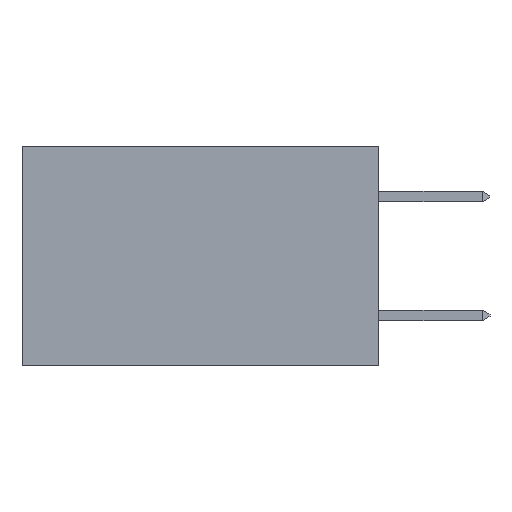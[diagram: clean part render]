
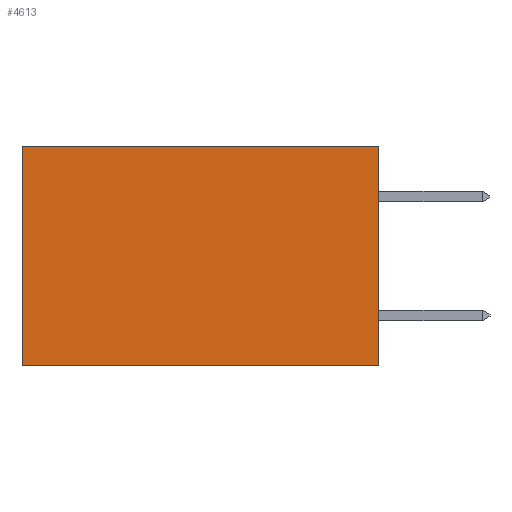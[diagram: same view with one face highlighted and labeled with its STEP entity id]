
A CAD part, left-side view. The second image highlights one B-rep face of the part: STEP entity #4613.
In plain terms, the highlighted planar face has unit normal (-1, 0, 0).
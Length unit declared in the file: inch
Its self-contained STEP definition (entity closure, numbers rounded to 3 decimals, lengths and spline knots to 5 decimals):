
#77 = ORIENTED_EDGE ( 'NONE', *, *, #442, .F. ) ;
#442 = EDGE_CURVE ( 'NONE', #3597, #3406, #8264, .T. ) ;
#462 = VECTOR ( 'NONE', #7460, 39.37008 ) ;
#479 = EDGE_CURVE ( 'NONE', #5677, #3597, #2644, .T. ) ;
#693 = EDGE_LOOP ( 'NONE', ( #6025, #77, #2320, #7729 ) ) ;
#2191 = DIRECTION ( 'NONE',  ( 0., 0., -1. ) ) ;
#2320 = ORIENTED_EDGE ( 'NONE', *, *, #479, .F. ) ;
#2624 = PLANE ( 'NONE',  #3133 ) ;
#2644 = LINE ( 'NONE', #6250, #462 ) ;
#3015 = CARTESIAN_POINT ( 'NONE',  ( 0.2615, 0., -0.37 ) ) ;
#3099 = VECTOR ( 'NONE', #6986, 39.37008 ) ;
#3106 = VECTOR ( 'NONE', #2191, 39.37008 ) ;
#3133 = AXIS2_PLACEMENT_3D ( 'NONE', #4029, #8460, #4862 ) ;
#3276 = DIRECTION ( 'NONE',  ( 0., 1., 0. ) ) ;
#3406 = VERTEX_POINT ( 'NONE', #4525 ) ;
#3597 = VERTEX_POINT ( 'NONE', #6735 ) ;
#4029 = CARTESIAN_POINT ( 'NONE',  ( 0.2615, 0., -0.37 ) ) ;
#4525 = CARTESIAN_POINT ( 'NONE',  ( 0.2615, 0.6, -0.37 ) ) ;
#4609 = EDGE_CURVE ( 'NONE', #5677, #4784, #7866, .T. ) ;
#4613 = ADVANCED_FACE ( 'NONE', ( #6178 ), #2624, .F. ) ;
#4682 = EDGE_CURVE ( 'NONE', #4784, #3406, #8437, .T. ) ;
#4730 = VECTOR ( 'NONE', #3276, 39.37008 ) ;
#4784 = VERTEX_POINT ( 'NONE', #7838 ) ;
#4862 = DIRECTION ( 'NONE',  ( 0., 0., -1. ) ) ;
#5444 = CARTESIAN_POINT ( 'NONE',  ( 0.2615, 0., 0. ) ) ;
#5677 = VERTEX_POINT ( 'NONE', #5444 ) ;
#5884 = CARTESIAN_POINT ( 'NONE',  ( 0.2615, 0.6, -0.37 ) ) ;
#6025 = ORIENTED_EDGE ( 'NONE', *, *, #4682, .T. ) ;
#6178 = FACE_OUTER_BOUND ( 'NONE', #693, .T. ) ;
#6250 = CARTESIAN_POINT ( 'NONE',  ( 0.2615, 0., -0.37 ) ) ;
#6735 = CARTESIAN_POINT ( 'NONE',  ( 0.2615, 0., -0.37 ) ) ;
#6986 = DIRECTION ( 'NONE',  ( 0., 1., 0. ) ) ;
#7460 = DIRECTION ( 'NONE',  ( 0., 0., -1. ) ) ;
#7729 = ORIENTED_EDGE ( 'NONE', *, *, #4609, .T. ) ;
#7838 = CARTESIAN_POINT ( 'NONE',  ( 0.2615, 0.6, 0. ) ) ;
#7866 = LINE ( 'NONE', #7920, #4730 ) ;
#7920 = CARTESIAN_POINT ( 'NONE',  ( 0.2615, 0., 0. ) ) ;
#8264 = LINE ( 'NONE', #3015, #3099 ) ;
#8437 = LINE ( 'NONE', #5884, #3106 ) ;
#8460 = DIRECTION ( 'NONE',  ( 1., 0., 0. ) ) ;
